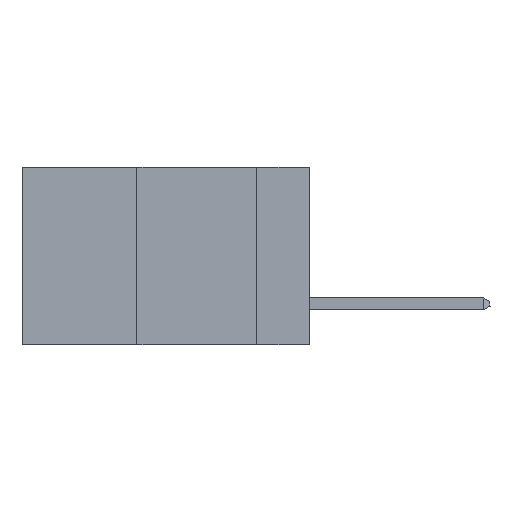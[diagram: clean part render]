
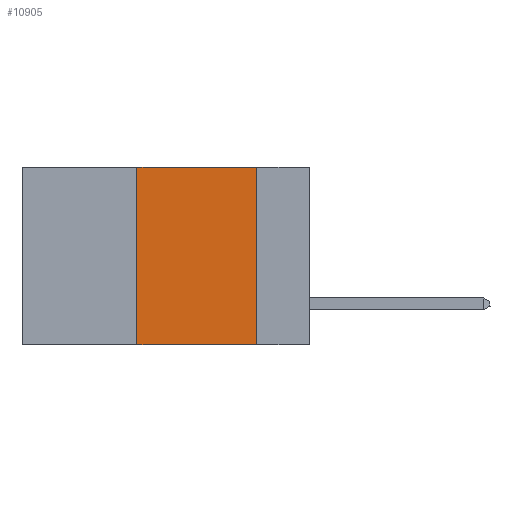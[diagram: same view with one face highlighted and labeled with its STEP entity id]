
A CAD part, left-side view. The second image highlights one B-rep face of the part: STEP entity #10905.
In plain terms, the highlighted planar face has unit normal (-1, 0, 0).
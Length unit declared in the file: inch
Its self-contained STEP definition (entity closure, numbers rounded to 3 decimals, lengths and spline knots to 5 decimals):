
#92 = CARTESIAN_POINT ( 'NONE',  ( 0., 0.36, -0.37 ) ) ;
#164 = DIRECTION ( 'NONE',  ( 1., 0., 0. ) ) ;
#1388 = ORIENTED_EDGE ( 'NONE', *, *, #8076, .F. ) ;
#1627 = VECTOR ( 'NONE', #14013, 39.37008 ) ;
#2618 = EDGE_CURVE ( 'NONE', #15343, #17513, #14338, .T. ) ;
#3392 = DIRECTION ( 'NONE',  ( 0., -1., 0. ) ) ;
#4342 = CARTESIAN_POINT ( 'NONE',  ( 0., 0.6, 0. ) ) ;
#4909 = CARTESIAN_POINT ( 'NONE',  ( 0., 0.36, 0. ) ) ;
#5034 = DIRECTION ( 'NONE',  ( 0., 0., 1. ) ) ;
#6040 = LINE ( 'NONE', #13314, #12658 ) ;
#7256 = EDGE_LOOP ( 'NONE', ( #17856, #9043, #1388, #7406 ) ) ;
#7406 = ORIENTED_EDGE ( 'NONE', *, *, #2618, .T. ) ;
#7964 = EDGE_CURVE ( 'NONE', #15264, #9224, #6040, .T. ) ;
#8076 = EDGE_CURVE ( 'NONE', #15343, #15264, #9982, .T. ) ;
#8530 = DIRECTION ( 'NONE',  ( 0., 0., -1. ) ) ;
#9043 = ORIENTED_EDGE ( 'NONE', *, *, #7964, .F. ) ;
#9224 = VERTEX_POINT ( 'NONE', #14572 ) ;
#9982 = LINE ( 'NONE', #16484, #18142 ) ;
#10004 = PLANE ( 'NONE',  #12930 ) ;
#10905 = ADVANCED_FACE ( 'NONE', ( #12558 ), #10004, .F. ) ;
#11237 = DIRECTION ( 'NONE',  ( 0., 0., -1. ) ) ;
#11408 = CARTESIAN_POINT ( 'NONE',  ( 0., 0.6, -0.37 ) ) ;
#11563 = LINE ( 'NONE', #14025, #14880 ) ;
#12558 = FACE_OUTER_BOUND ( 'NONE', #7256, .T. ) ;
#12658 = VECTOR ( 'NONE', #3392, 39.37008 ) ;
#12930 = AXIS2_PLACEMENT_3D ( 'NONE', #4342, #164, #11237 ) ;
#13314 = CARTESIAN_POINT ( 'NONE',  ( 0., 0.6, 0. ) ) ;
#13683 = EDGE_CURVE ( 'NONE', #9224, #17513, #11563, .T. ) ;
#14013 = DIRECTION ( 'NONE',  ( 0., -1., 0. ) ) ;
#14025 = CARTESIAN_POINT ( 'NONE',  ( 0., 0.11, 0. ) ) ;
#14338 = LINE ( 'NONE', #11408, #1627 ) ;
#14572 = CARTESIAN_POINT ( 'NONE',  ( 0., 0.11, 0. ) ) ;
#14880 = VECTOR ( 'NONE', #8530, 39.37008 ) ;
#15264 = VERTEX_POINT ( 'NONE', #4909 ) ;
#15343 = VERTEX_POINT ( 'NONE', #92 ) ;
#16174 = CARTESIAN_POINT ( 'NONE',  ( 0., 0.11, -0.37 ) ) ;
#16484 = CARTESIAN_POINT ( 'NONE',  ( 0., 0.36, 0. ) ) ;
#17513 = VERTEX_POINT ( 'NONE', #16174 ) ;
#17856 = ORIENTED_EDGE ( 'NONE', *, *, #13683, .F. ) ;
#18142 = VECTOR ( 'NONE', #5034, 39.37008 ) ;
